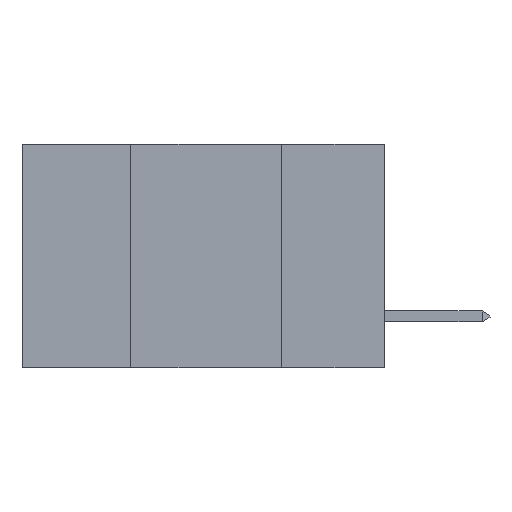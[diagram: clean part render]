
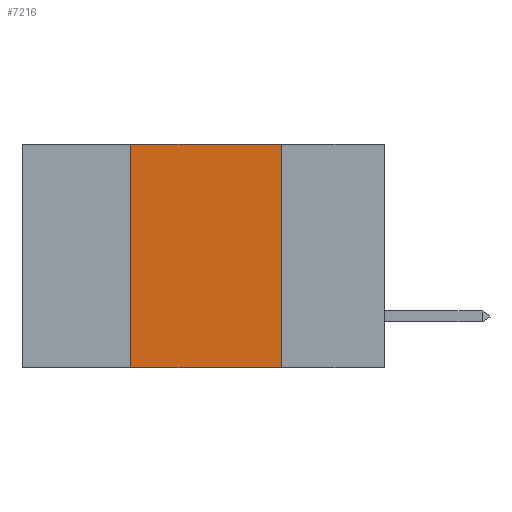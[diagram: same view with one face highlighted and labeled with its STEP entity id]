
A CAD part, left-side view. The second image highlights one B-rep face of the part: STEP entity #7216.
In plain terms, the highlighted planar face has unit normal (-1, 0, 0).
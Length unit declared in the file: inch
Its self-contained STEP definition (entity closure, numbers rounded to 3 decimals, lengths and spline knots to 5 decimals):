
#1053 = VERTEX_POINT ( 'NONE', #29993 ) ;
#3112 = LINE ( 'NONE', #27383, #19794 ) ;
#4315 = VERTEX_POINT ( 'NONE', #30567 ) ;
#4896 = EDGE_CURVE ( 'NONE', #4315, #1053, #7444, .T. ) ;
#6500 = LINE ( 'NONE', #27832, #40622 ) ;
#6788 = DIRECTION ( 'NONE',  ( 1., 0., 0. ) ) ;
#7117 = CARTESIAN_POINT ( 'NONE',  ( 0., 0.42, 0. ) ) ;
#7216 = ADVANCED_FACE ( 'NONE', ( #39202 ), #20021, .F. ) ;
#7444 = LINE ( 'NONE', #7117, #41578 ) ;
#8850 = ORIENTED_EDGE ( 'NONE', *, *, #16094, .F. ) ;
#10421 = DIRECTION ( 'NONE',  ( 0., 0., 1. ) ) ;
#12328 = LINE ( 'NONE', #29276, #29035 ) ;
#14860 = CARTESIAN_POINT ( 'NONE',  ( 0., 0.17, 0. ) ) ;
#14920 = ORIENTED_EDGE ( 'NONE', *, *, #32808, .T. ) ;
#16094 = EDGE_CURVE ( 'NONE', #1053, #37734, #12328, .T. ) ;
#18169 = ORIENTED_EDGE ( 'NONE', *, *, #4896, .F. ) ;
#18461 = VERTEX_POINT ( 'NONE', #38637 ) ;
#19785 = EDGE_LOOP ( 'NONE', ( #20336, #8850, #18169, #14920 ) ) ;
#19794 = VECTOR ( 'NONE', #30678, 39.37008 ) ;
#20021 = PLANE ( 'NONE',  #29190 ) ;
#20336 = ORIENTED_EDGE ( 'NONE', *, *, #34943, .F. ) ;
#27383 = CARTESIAN_POINT ( 'NONE',  ( 0., 0.17, 0. ) ) ;
#27832 = CARTESIAN_POINT ( 'NONE',  ( 0., 0.6, -0.37 ) ) ;
#29035 = VECTOR ( 'NONE', #29144, 39.37008 ) ;
#29144 = DIRECTION ( 'NONE',  ( 0., -1., 0. ) ) ;
#29190 = AXIS2_PLACEMENT_3D ( 'NONE', #36453, #6788, #30050 ) ;
#29276 = CARTESIAN_POINT ( 'NONE',  ( 0., 0.6, 0. ) ) ;
#29993 = CARTESIAN_POINT ( 'NONE',  ( 0., 0.42, 0. ) ) ;
#30050 = DIRECTION ( 'NONE',  ( 0., 0., -1. ) ) ;
#30567 = CARTESIAN_POINT ( 'NONE',  ( 0., 0.42, -0.37 ) ) ;
#30678 = DIRECTION ( 'NONE',  ( 0., 0., -1. ) ) ;
#32808 = EDGE_CURVE ( 'NONE', #4315, #18461, #6500, .T. ) ;
#34943 = EDGE_CURVE ( 'NONE', #37734, #18461, #3112, .T. ) ;
#36453 = CARTESIAN_POINT ( 'NONE',  ( 0., 0.6, 0. ) ) ;
#37734 = VERTEX_POINT ( 'NONE', #14860 ) ;
#38637 = CARTESIAN_POINT ( 'NONE',  ( 0., 0.17, -0.37 ) ) ;
#39202 = FACE_OUTER_BOUND ( 'NONE', #19785, .T. ) ;
#40622 = VECTOR ( 'NONE', #40674, 39.37008 ) ;
#40674 = DIRECTION ( 'NONE',  ( 0., -1., 0. ) ) ;
#41578 = VECTOR ( 'NONE', #10421, 39.37008 ) ;
